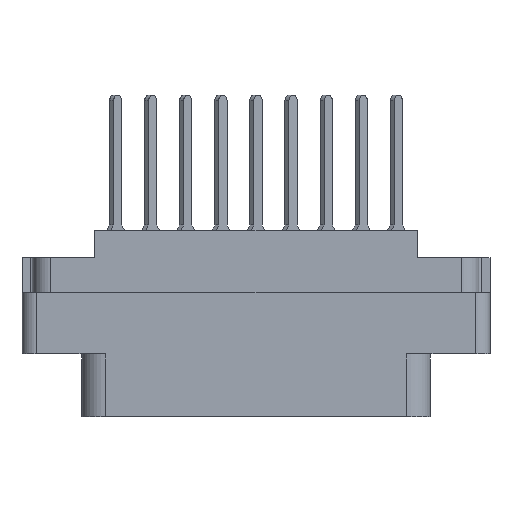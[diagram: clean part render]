
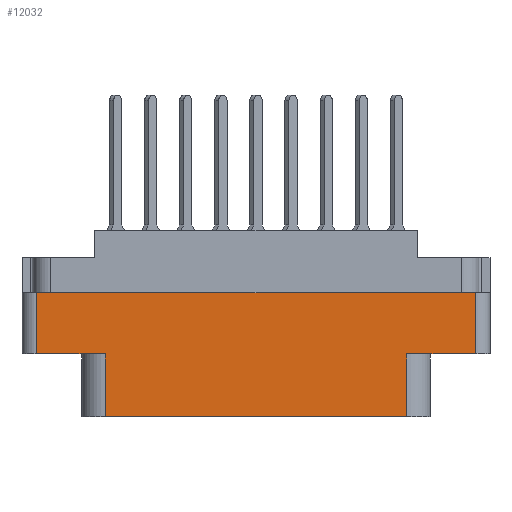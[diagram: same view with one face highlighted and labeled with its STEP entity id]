
A CAD part, front view. The second image highlights one B-rep face of the part: STEP entity #12032.
In plain terms, the highlighted planar face has unit normal (0, -1, 0).
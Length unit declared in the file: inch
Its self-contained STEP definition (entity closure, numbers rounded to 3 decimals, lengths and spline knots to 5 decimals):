
#240 = VERTEX_POINT ( 'NONE', #10427 ) ;
#459 = ORIENTED_EDGE ( 'NONE', *, *, #19940, .T. ) ;
#824 = DIRECTION ( 'NONE',  ( 1., 0., 0. ) ) ;
#1518 = LINE ( 'NONE', #26078, #3676 ) ;
#2029 = VERTEX_POINT ( 'NONE', #14923 ) ;
#3167 = VECTOR ( 'NONE', #29472, 39.37008 ) ;
#3213 = CARTESIAN_POINT ( 'NONE',  ( -0.938, -0.438, -0.798 ) ) ;
#3568 = CARTESIAN_POINT ( 'NONE',  ( -1., -0.438, -0.268 ) ) ;
#3676 = VECTOR ( 'NONE', #9135, 39.37008 ) ;
#3837 = EDGE_CURVE ( 'NONE', #31821, #2029, #1518, .T. ) ;
#4390 = ORIENTED_EDGE ( 'NONE', *, *, #3837, .F. ) ;
#4728 = VECTOR ( 'NONE', #24314, 39.37008 ) ;
#6297 = CARTESIAN_POINT ( 'NONE',  ( -0.938, -0.438, -0.798 ) ) ;
#6946 = VERTEX_POINT ( 'NONE', #18255 ) ;
#8419 = CARTESIAN_POINT ( 'NONE',  ( 0.938, -0.438, -0.268 ) ) ;
#8517 = VECTOR ( 'NONE', #31603, 39.37008 ) ;
#9135 = DIRECTION ( 'NONE',  ( -1., 0., 0. ) ) ;
#9341 = VERTEX_POINT ( 'NONE', #33841 ) ;
#9614 = CARTESIAN_POINT ( 'NONE',  ( 0.938, -0.438, -0.529 ) ) ;
#9667 = VECTOR ( 'NONE', #10277, 39.37008 ) ;
#10277 = DIRECTION ( 'NONE',  ( 0., 0., 1. ) ) ;
#10427 = CARTESIAN_POINT ( 'NONE',  ( -0.938, -0.438, -0.268 ) ) ;
#10584 = LINE ( 'NONE', #35503, #9667 ) ;
#11085 = EDGE_CURVE ( 'NONE', #27159, #240, #11576, .T. ) ;
#11522 = ORIENTED_EDGE ( 'NONE', *, *, #21158, .F. ) ;
#11576 = LINE ( 'NONE', #21105, #3167 ) ;
#11681 = EDGE_CURVE ( 'NONE', #27159, #9341, #27450, .T. ) ;
#12032 = ADVANCED_FACE ( 'NONE', ( #23407 ), #17280, .T. ) ;
#12153 = CARTESIAN_POINT ( 'NONE',  ( -0.938, -0.438, -0.529 ) ) ;
#12514 = AXIS2_PLACEMENT_3D ( 'NONE', #3213, #25686, #34105 ) ;
#14014 = ORIENTED_EDGE ( 'NONE', *, *, #18715, .T. ) ;
#14426 = ORIENTED_EDGE ( 'NONE', *, *, #21734, .T. ) ;
#14923 = CARTESIAN_POINT ( 'NONE',  ( 0.644, -0.438, -0.529 ) ) ;
#14983 = CARTESIAN_POINT ( 'NONE',  ( 0., -0.438, -0.529 ) ) ;
#15161 = LINE ( 'NONE', #3568, #8517 ) ;
#15789 = LINE ( 'NONE', #27188, #4728 ) ;
#16990 = CARTESIAN_POINT ( 'NONE',  ( 0.644, -0.438, -0.798 ) ) ;
#17218 = EDGE_CURVE ( 'NONE', #240, #25019, #15161, .T. ) ;
#17280 = PLANE ( 'NONE',  #12514 ) ;
#17696 = ORIENTED_EDGE ( 'NONE', *, *, #17218, .F. ) ;
#18255 = CARTESIAN_POINT ( 'NONE',  ( -0.644, -0.438, -0.798 ) ) ;
#18696 = ORIENTED_EDGE ( 'NONE', *, *, #11085, .F. ) ;
#18715 = EDGE_CURVE ( 'NONE', #6946, #18985, #22970, .T. ) ;
#18985 = VERTEX_POINT ( 'NONE', #16990 ) ;
#19918 = VECTOR ( 'NONE', #31272, 39.37008 ) ;
#19940 = EDGE_CURVE ( 'NONE', #31821, #25019, #10584, .T. ) ;
#21105 = CARTESIAN_POINT ( 'NONE',  ( -0.938, -0.438, -0.798 ) ) ;
#21158 = EDGE_CURVE ( 'NONE', #2029, #18985, #33048, .T. ) ;
#21734 = EDGE_CURVE ( 'NONE', #9341, #6946, #15789, .T. ) ;
#22970 = LINE ( 'NONE', #6297, #19918 ) ;
#23407 = FACE_OUTER_BOUND ( 'NONE', #28448, .T. ) ;
#24314 = DIRECTION ( 'NONE',  ( 0., 0., -1. ) ) ;
#25019 = VERTEX_POINT ( 'NONE', #8419 ) ;
#25686 = DIRECTION ( 'NONE',  ( 0., -1., 0. ) ) ;
#26078 = CARTESIAN_POINT ( 'NONE',  ( 0., -0.438, -0.529 ) ) ;
#27159 = VERTEX_POINT ( 'NONE', #12153 ) ;
#27188 = CARTESIAN_POINT ( 'NONE',  ( -0.644, -0.438, -0.529 ) ) ;
#27450 = LINE ( 'NONE', #14983, #34083 ) ;
#28448 = EDGE_LOOP ( 'NONE', ( #14426, #14014, #11522, #4390, #459, #17696, #18696, #34136 ) ) ;
#29472 = DIRECTION ( 'NONE',  ( 0., 0., 1. ) ) ;
#29738 = DIRECTION ( 'NONE',  ( 0., 0., -1. ) ) ;
#31272 = DIRECTION ( 'NONE',  ( 1., 0., 0. ) ) ;
#31603 = DIRECTION ( 'NONE',  ( 1., 0., 0. ) ) ;
#31727 = CARTESIAN_POINT ( 'NONE',  ( 0.644, -0.438, -0.529 ) ) ;
#31821 = VERTEX_POINT ( 'NONE', #9614 ) ;
#33048 = LINE ( 'NONE', #31727, #36575 ) ;
#33841 = CARTESIAN_POINT ( 'NONE',  ( -0.644, -0.438, -0.529 ) ) ;
#34083 = VECTOR ( 'NONE', #824, 39.37008 ) ;
#34105 = DIRECTION ( 'NONE',  ( 0., 0., -1. ) ) ;
#34136 = ORIENTED_EDGE ( 'NONE', *, *, #11681, .T. ) ;
#35503 = CARTESIAN_POINT ( 'NONE',  ( 0.938, -0.438, -0.798 ) ) ;
#36575 = VECTOR ( 'NONE', #29738, 39.37008 ) ;
